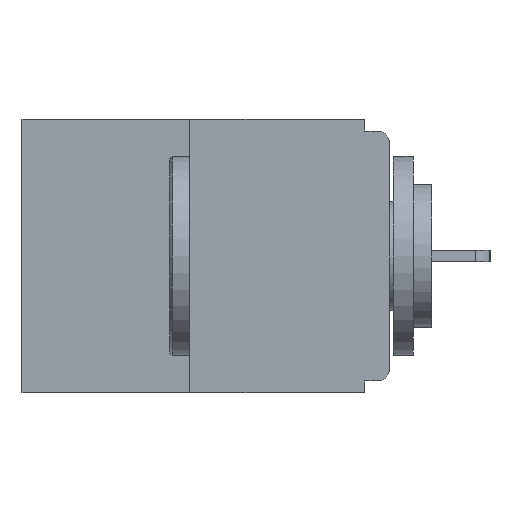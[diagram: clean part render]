
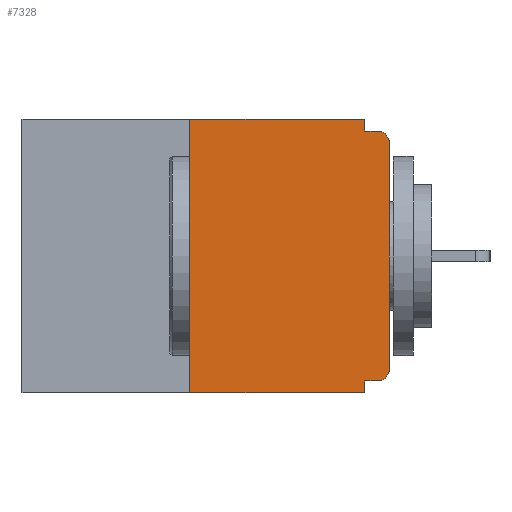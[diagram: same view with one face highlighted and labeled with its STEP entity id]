
A CAD part, left-side view. The second image highlights one B-rep face of the part: STEP entity #7328.
In plain terms, the highlighted planar face has unit normal (-1, 0, 0).
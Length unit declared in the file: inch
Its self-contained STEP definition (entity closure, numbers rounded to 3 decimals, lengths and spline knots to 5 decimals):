
#300 = AXIS2_PLACEMENT_3D ( 'NONE', #2745, #2738, #2713 ) ;
#379 = CARTESIAN_POINT ( 'NONE',  ( 0., 0., -0.015 ) ) ;
#487 = VERTEX_POINT ( 'NONE', #1362 ) ;
#675 = LINE ( 'NONE', #13117, #9098 ) ;
#772 = FACE_OUTER_BOUND ( 'NONE', #11014, .T. ) ;
#1142 = LINE ( 'NONE', #13786, #17876 ) ;
#1326 = VERTEX_POINT ( 'NONE', #20482 ) ;
#1362 = CARTESIAN_POINT ( 'NONE',  ( 0., 0.25, 0. ) ) ;
#1774 = CIRCLE ( 'NONE', #300, 0.015 ) ;
#1786 = CARTESIAN_POINT ( 'NONE',  ( 0., 0.46, 0. ) ) ;
#2136 = CARTESIAN_POINT ( 'NONE',  ( 0., 0.031, -0.015 ) ) ;
#2704 = CARTESIAN_POINT ( 'NONE',  ( 0., 0., -0.328 ) ) ;
#2713 = DIRECTION ( 'NONE',  ( 0., 0., -1. ) ) ;
#2738 = DIRECTION ( 'NONE',  ( -1., 0., 0. ) ) ;
#2745 = CARTESIAN_POINT ( 'NONE',  ( 0., 0.015, -0.03 ) ) ;
#3292 = CARTESIAN_POINT ( 'NONE',  ( 0., 0., -0.313 ) ) ;
#3313 = VERTEX_POINT ( 'NONE', #10178 ) ;
#3527 = DIRECTION ( 'NONE',  ( 0., -1., 0. ) ) ;
#3569 = VECTOR ( 'NONE', #3527, 39.37008 ) ;
#3606 = VERTEX_POINT ( 'NONE', #15142 ) ;
#3653 = ORIENTED_EDGE ( 'NONE', *, *, #9420, .T. ) ;
#3719 = VECTOR ( 'NONE', #20593, 39.37008 ) ;
#3821 = VECTOR ( 'NONE', #19141, 39.37008 ) ;
#4103 = DIRECTION ( 'NONE',  ( 0., 0., -1. ) ) ;
#4397 = VERTEX_POINT ( 'NONE', #3292 ) ;
#5365 = AXIS2_PLACEMENT_3D ( 'NONE', #18883, #9463, #20396 ) ;
#5670 = LINE ( 'NONE', #379, #19344 ) ;
#6474 = VERTEX_POINT ( 'NONE', #14033 ) ;
#6566 = ORIENTED_EDGE ( 'NONE', *, *, #6910, .T. ) ;
#6910 = EDGE_CURVE ( 'NONE', #3313, #13414, #8208, .T. ) ;
#7104 = VERTEX_POINT ( 'NONE', #18062 ) ;
#7328 = ADVANCED_FACE ( 'NONE', ( #772 ), #15375, .F. ) ;
#8208 = LINE ( 'NONE', #20591, #3719 ) ;
#9057 = VECTOR ( 'NONE', #17251, 39.37008 ) ;
#9098 = VECTOR ( 'NONE', #11590, 39.37008 ) ;
#9420 = EDGE_CURVE ( 'NONE', #7104, #3606, #1774, .T. ) ;
#9463 = DIRECTION ( 'NONE',  ( -1., 0., 0. ) ) ;
#9464 = CARTESIAN_POINT ( 'NONE',  ( 0., 0.25, 0. ) ) ;
#9863 = ORIENTED_EDGE ( 'NONE', *, *, #19192, .F. ) ;
#9914 = EDGE_CURVE ( 'NONE', #3313, #487, #12809, .T. ) ;
#10178 = CARTESIAN_POINT ( 'NONE',  ( 0., 0.25, -0.343 ) ) ;
#10346 = DIRECTION ( 'NONE',  ( 0., -1., 0. ) ) ;
#10721 = EDGE_CURVE ( 'NONE', #4397, #7104, #675, .T. ) ;
#11014 = EDGE_LOOP ( 'NONE', ( #9863, #14546, #6566, #15540, #19685, #11802, #20160, #3653, #12320, #16506 ) ) ;
#11511 = EDGE_CURVE ( 'NONE', #12286, #15145, #1142, .T. ) ;
#11590 = DIRECTION ( 'NONE',  ( 0., 0., 1. ) ) ;
#11780 = EDGE_CURVE ( 'NONE', #1326, #13414, #12472, .T. ) ;
#11802 = ORIENTED_EDGE ( 'NONE', *, *, #13615, .T. ) ;
#12242 = LINE ( 'NONE', #1786, #3569 ) ;
#12286 = VERTEX_POINT ( 'NONE', #18362 ) ;
#12320 = ORIENTED_EDGE ( 'NONE', *, *, #19916, .F. ) ;
#12472 = LINE ( 'NONE', #14467, #3821 ) ;
#12809 = LINE ( 'NONE', #9464, #13297 ) ;
#13117 = CARTESIAN_POINT ( 'NONE',  ( 0., 0., 0. ) ) ;
#13297 = VECTOR ( 'NONE', #14134, 39.37008 ) ;
#13414 = VERTEX_POINT ( 'NONE', #15238 ) ;
#13615 = EDGE_CURVE ( 'NONE', #6474, #4397, #15120, .T. ) ;
#13715 = LINE ( 'NONE', #2704, #9057 ) ;
#13786 = CARTESIAN_POINT ( 'NONE',  ( 0., 0.031, 0. ) ) ;
#14033 = CARTESIAN_POINT ( 'NONE',  ( 0., 0.015, -0.328 ) ) ;
#14134 = DIRECTION ( 'NONE',  ( 0., 0., 1. ) ) ;
#14467 = CARTESIAN_POINT ( 'NONE',  ( 0., 0.031, -0.343 ) ) ;
#14546 = ORIENTED_EDGE ( 'NONE', *, *, #9914, .F. ) ;
#15120 = CIRCLE ( 'NONE', #5365, 0.015 ) ;
#15142 = CARTESIAN_POINT ( 'NONE',  ( 0., 0.015, -0.015 ) ) ;
#15145 = VERTEX_POINT ( 'NONE', #2136 ) ;
#15193 = DIRECTION ( 'NONE',  ( 0., 0., -1. ) ) ;
#15233 = DIRECTION ( 'NONE',  ( 1., 0., 0. ) ) ;
#15238 = CARTESIAN_POINT ( 'NONE',  ( 0., 0.031, -0.343 ) ) ;
#15277 = CARTESIAN_POINT ( 'NONE',  ( 0., 0.46, 0. ) ) ;
#15375 = PLANE ( 'NONE',  #18778 ) ;
#15540 = ORIENTED_EDGE ( 'NONE', *, *, #11780, .F. ) ;
#16506 = ORIENTED_EDGE ( 'NONE', *, *, #11511, .F. ) ;
#17251 = DIRECTION ( 'NONE',  ( 0., 1., 0. ) ) ;
#17876 = VECTOR ( 'NONE', #4103, 39.37008 ) ;
#18062 = CARTESIAN_POINT ( 'NONE',  ( 0., 0., -0.03 ) ) ;
#18362 = CARTESIAN_POINT ( 'NONE',  ( 0., 0.031, 0. ) ) ;
#18778 = AXIS2_PLACEMENT_3D ( 'NONE', #15277, #15233, #15193 ) ;
#18883 = CARTESIAN_POINT ( 'NONE',  ( 0., 0.015, -0.313 ) ) ;
#19141 = DIRECTION ( 'NONE',  ( 0., 0., -1. ) ) ;
#19192 = EDGE_CURVE ( 'NONE', #487, #12286, #12242, .T. ) ;
#19344 = VECTOR ( 'NONE', #10346, 39.37008 ) ;
#19536 = EDGE_CURVE ( 'NONE', #6474, #1326, #13715, .T. ) ;
#19685 = ORIENTED_EDGE ( 'NONE', *, *, #19536, .F. ) ;
#19916 = EDGE_CURVE ( 'NONE', #15145, #3606, #5670, .T. ) ;
#20160 = ORIENTED_EDGE ( 'NONE', *, *, #10721, .T. ) ;
#20396 = DIRECTION ( 'NONE',  ( 0., 0., -1. ) ) ;
#20482 = CARTESIAN_POINT ( 'NONE',  ( 0., 0.031, -0.328 ) ) ;
#20591 = CARTESIAN_POINT ( 'NONE',  ( 0., 0.46, -0.343 ) ) ;
#20593 = DIRECTION ( 'NONE',  ( 0., -1., 0. ) ) ;
